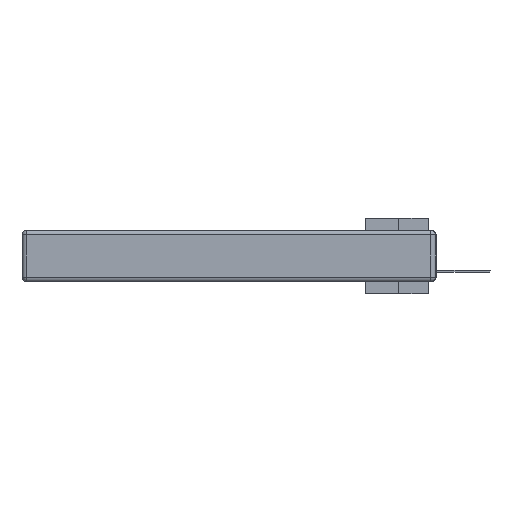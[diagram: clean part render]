
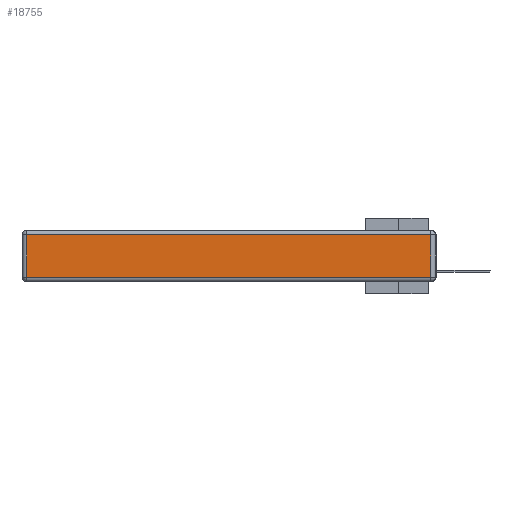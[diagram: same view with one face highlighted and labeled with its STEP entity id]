
A CAD part, left-side view. The second image highlights one B-rep face of the part: STEP entity #18755.
In plain terms, the highlighted planar face has unit normal (-1, 0, 0).
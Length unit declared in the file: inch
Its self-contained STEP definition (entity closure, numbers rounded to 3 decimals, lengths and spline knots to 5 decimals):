
#310 = CARTESIAN_POINT ( 'NONE',  ( 0., 0., -0.313 ) ) ;
#545 = DIRECTION ( 'NONE',  ( 0., -1., 0. ) ) ;
#752 = CARTESIAN_POINT ( 'NONE',  ( 0., 2.72, -0.313 ) ) ;
#902 = ORIENTED_EDGE ( 'NONE', *, *, #1986, .T. ) ;
#1084 = EDGE_LOOP ( 'NONE', ( #6649, #33757, #14350, #902 ) ) ;
#1986 = EDGE_CURVE ( 'NONE', #13763, #23353, #22335, .T. ) ;
#3456 = CARTESIAN_POINT ( 'NONE',  ( 0., 0.03, -0.313 ) ) ;
#6649 = ORIENTED_EDGE ( 'NONE', *, *, #34325, .T. ) ;
#7181 = DIRECTION ( 'NONE',  ( 0., 1., 0. ) ) ;
#7319 = CARTESIAN_POINT ( 'NONE',  ( 0., 2.75, -0.03 ) ) ;
#7717 = CARTESIAN_POINT ( 'NONE',  ( 0., 0.03, -0.03 ) ) ;
#11066 = DIRECTION ( 'NONE',  ( 0., 0., 1. ) ) ;
#12841 = EDGE_CURVE ( 'NONE', #28669, #33118, #19799, .T. ) ;
#13101 = DIRECTION ( 'NONE',  ( -1., 0., 0. ) ) ;
#13225 = PLANE ( 'NONE',  #14804 ) ;
#13763 = VERTEX_POINT ( 'NONE', #19177 ) ;
#14350 = ORIENTED_EDGE ( 'NONE', *, *, #29364, .T. ) ;
#14445 = VECTOR ( 'NONE', #7181, 39.37008 ) ;
#14804 = AXIS2_PLACEMENT_3D ( 'NONE', #32904, #13101, #15703 ) ;
#15703 = DIRECTION ( 'NONE',  ( 0., 0., 1. ) ) ;
#18455 = LINE ( 'NONE', #7319, #14445 ) ;
#18585 = CARTESIAN_POINT ( 'NONE',  ( 0., 2.72, -0.343 ) ) ;
#18705 = DIRECTION ( 'NONE',  ( 0., 0., -1. ) ) ;
#18755 = ADVANCED_FACE ( 'NONE', ( #27567 ), #13225, .T. ) ;
#19177 = CARTESIAN_POINT ( 'NONE',  ( 0., 2.72, -0.03 ) ) ;
#19799 = LINE ( 'NONE', #22603, #31584 ) ;
#21324 = VECTOR ( 'NONE', #545, 39.37008 ) ;
#22335 = LINE ( 'NONE', #18585, #24118 ) ;
#22603 = CARTESIAN_POINT ( 'NONE',  ( 0., 0.03, -0.343 ) ) ;
#23353 = VERTEX_POINT ( 'NONE', #752 ) ;
#24118 = VECTOR ( 'NONE', #18705, 39.37008 ) ;
#27567 = FACE_OUTER_BOUND ( 'NONE', #1084, .T. ) ;
#28669 = VERTEX_POINT ( 'NONE', #3456 ) ;
#29292 = LINE ( 'NONE', #310, #21324 ) ;
#29364 = EDGE_CURVE ( 'NONE', #33118, #13763, #18455, .T. ) ;
#31584 = VECTOR ( 'NONE', #11066, 39.37008 ) ;
#32904 = CARTESIAN_POINT ( 'NONE',  ( 0., 0., -0.343 ) ) ;
#33118 = VERTEX_POINT ( 'NONE', #7717 ) ;
#33757 = ORIENTED_EDGE ( 'NONE', *, *, #12841, .T. ) ;
#34325 = EDGE_CURVE ( 'NONE', #23353, #28669, #29292, .T. ) ;
